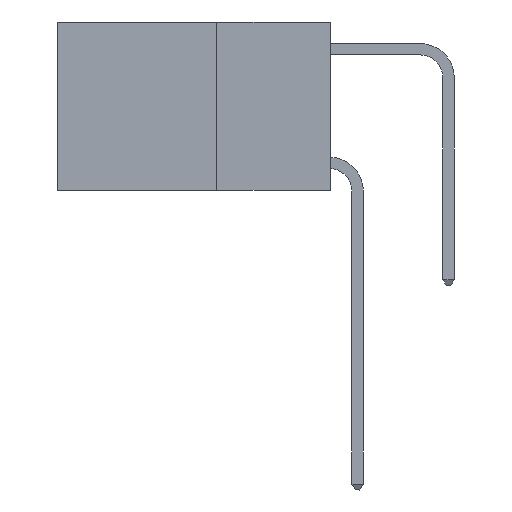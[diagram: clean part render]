
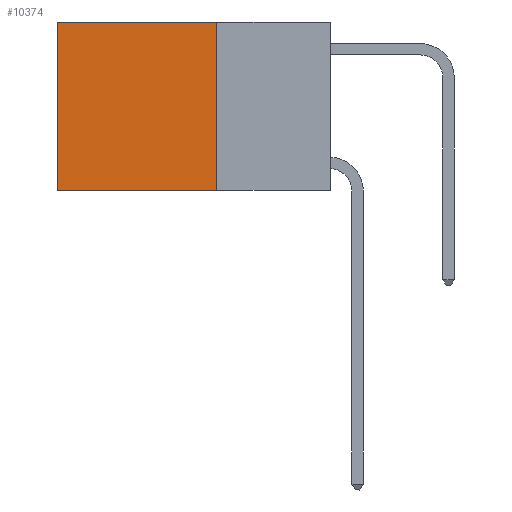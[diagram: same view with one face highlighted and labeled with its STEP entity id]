
A CAD part, left-side view. The second image highlights one B-rep face of the part: STEP entity #10374.
In plain terms, the highlighted planar face has unit normal (-1, 0, 0).
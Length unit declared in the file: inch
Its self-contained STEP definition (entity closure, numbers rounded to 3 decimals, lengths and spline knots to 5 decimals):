
#261 = VERTEX_POINT ( 'NONE', #9818 ) ;
#405 = DIRECTION ( 'NONE',  ( 0., 0., -1. ) ) ;
#1631 = DIRECTION ( 'NONE',  ( 0., 1., 0. ) ) ;
#1693 = EDGE_CURVE ( 'NONE', #8328, #6848, #14496, .T. ) ;
#2079 = ORIENTED_EDGE ( 'NONE', *, *, #1693, .F. ) ;
#2928 = CARTESIAN_POINT ( 'NONE',  ( 0.2625, 0.25, 0. ) ) ;
#3087 = CARTESIAN_POINT ( 'NONE',  ( 0.2625, 0.6, 0. ) ) ;
#3650 = CARTESIAN_POINT ( 'NONE',  ( 0.2625, 0.25, 0. ) ) ;
#3719 = FACE_OUTER_BOUND ( 'NONE', #4877, .T. ) ;
#3777 = LINE ( 'NONE', #3087, #10139 ) ;
#3978 = LINE ( 'NONE', #2928, #5299 ) ;
#4300 = DIRECTION ( 'NONE',  ( 0., 0., -1. ) ) ;
#4877 = EDGE_LOOP ( 'NONE', ( #5044, #2079, #14519, #8724 ) ) ;
#5044 = ORIENTED_EDGE ( 'NONE', *, *, #9843, .T. ) ;
#5159 = CARTESIAN_POINT ( 'NONE',  ( 0.2625, 0.6, -0.37 ) ) ;
#5192 = LINE ( 'NONE', #8967, #12897 ) ;
#5299 = VECTOR ( 'NONE', #14793, 39.37008 ) ;
#6848 = VERTEX_POINT ( 'NONE', #5159 ) ;
#7287 = DIRECTION ( 'NONE',  ( 1., 0., 0. ) ) ;
#7355 = VERTEX_POINT ( 'NONE', #11905 ) ;
#8328 = VERTEX_POINT ( 'NONE', #14690 ) ;
#8360 = EDGE_CURVE ( 'NONE', #261, #7355, #5192, .T. ) ;
#8724 = ORIENTED_EDGE ( 'NONE', *, *, #8360, .T. ) ;
#8967 = CARTESIAN_POINT ( 'NONE',  ( 0.2625, 0.25, 0. ) ) ;
#9818 = CARTESIAN_POINT ( 'NONE',  ( 0.2625, 0.25, 0. ) ) ;
#9843 = EDGE_CURVE ( 'NONE', #7355, #6848, #3777, .T. ) ;
#10139 = VECTOR ( 'NONE', #4300, 39.37008 ) ;
#10374 = ADVANCED_FACE ( 'NONE', ( #3719 ), #10663, .F. ) ;
#10663 = PLANE ( 'NONE',  #14746 ) ;
#11905 = CARTESIAN_POINT ( 'NONE',  ( 0.2625, 0.6, 0. ) ) ;
#11991 = VECTOR ( 'NONE', #1631, 39.37008 ) ;
#12897 = VECTOR ( 'NONE', #13417, 39.37008 ) ;
#13321 = CARTESIAN_POINT ( 'NONE',  ( 0.2625, 0.25, -0.37 ) ) ;
#13417 = DIRECTION ( 'NONE',  ( 0., 1., 0. ) ) ;
#13968 = EDGE_CURVE ( 'NONE', #261, #8328, #3978, .T. ) ;
#14496 = LINE ( 'NONE', #13321, #11991 ) ;
#14519 = ORIENTED_EDGE ( 'NONE', *, *, #13968, .F. ) ;
#14690 = CARTESIAN_POINT ( 'NONE',  ( 0.2625, 0.25, -0.37 ) ) ;
#14746 = AXIS2_PLACEMENT_3D ( 'NONE', #3650, #7287, #405 ) ;
#14793 = DIRECTION ( 'NONE',  ( 0., 0., -1. ) ) ;
